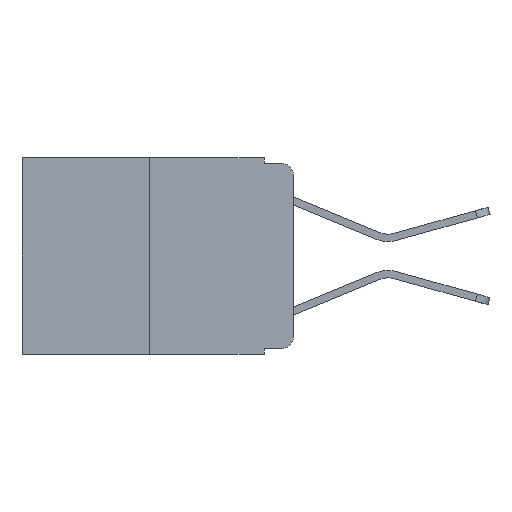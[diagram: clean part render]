
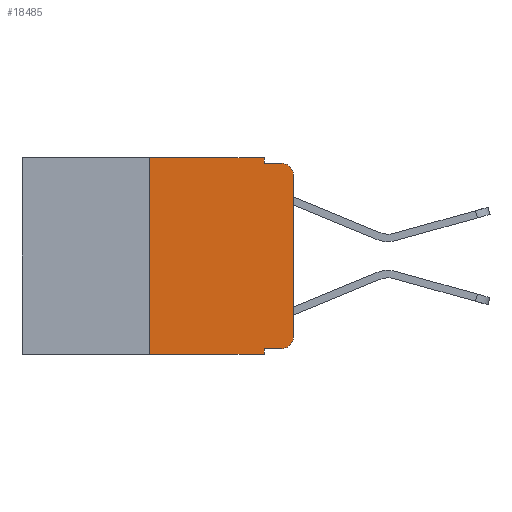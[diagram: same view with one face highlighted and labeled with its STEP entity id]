
A CAD part, left-side view. The second image highlights one B-rep face of the part: STEP entity #18485.
In plain terms, the highlighted planar face has unit normal (-1, 0, 0).
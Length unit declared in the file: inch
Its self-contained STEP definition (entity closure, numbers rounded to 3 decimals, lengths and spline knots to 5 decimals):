
#162 = VECTOR ( 'NONE', #13785, 39.37008 ) ;
#295 = VECTOR ( 'NONE', #14769, 39.37008 ) ;
#560 = VERTEX_POINT ( 'NONE', #21218 ) ;
#864 = EDGE_CURVE ( 'NONE', #19820, #19626, #5667, .T. ) ;
#1301 = LINE ( 'NONE', #9719, #11378 ) ;
#1340 = CARTESIAN_POINT ( 'NONE',  ( 0., 0.051, 0. ) ) ;
#1882 = CARTESIAN_POINT ( 'NONE',  ( 0., 0.051, -0.333 ) ) ;
#2022 = VERTEX_POINT ( 'NONE', #6495 ) ;
#2141 = DIRECTION ( 'NONE',  ( 0., -1., 0. ) ) ;
#2191 = LINE ( 'NONE', #12164, #6284 ) ;
#2541 = AXIS2_PLACEMENT_3D ( 'NONE', #8536, #4469, #12557 ) ;
#3460 = CARTESIAN_POINT ( 'NONE',  ( 0., 0., 0. ) ) ;
#3490 = CARTESIAN_POINT ( 'NONE',  ( 0., 0.25, 0. ) ) ;
#3797 = CARTESIAN_POINT ( 'NONE',  ( 0., 0.051, -0.333 ) ) ;
#3798 = LINE ( 'NONE', #20362, #19010 ) ;
#4059 = LINE ( 'NONE', #1340, #8797 ) ;
#4469 = DIRECTION ( 'NONE',  ( 1., 0., 0. ) ) ;
#4685 = DIRECTION ( 'NONE',  ( 0., -1., 0. ) ) ;
#4912 = EDGE_CURVE ( 'NONE', #14279, #19626, #21799, .T. ) ;
#5306 = FACE_OUTER_BOUND ( 'NONE', #12608, .T. ) ;
#5667 = LINE ( 'NONE', #18038, #295 ) ;
#6263 = EDGE_CURVE ( 'NONE', #2022, #14279, #9125, .T. ) ;
#6284 = VECTOR ( 'NONE', #2141, 39.37008 ) ;
#6495 = CARTESIAN_POINT ( 'NONE',  ( 0., 0., -0.313 ) ) ;
#7077 = CARTESIAN_POINT ( 'NONE',  ( 0., 0.02, -0.333 ) ) ;
#7166 = ORIENTED_EDGE ( 'NONE', *, *, #18697, .T. ) ;
#7593 = DIRECTION ( 'NONE',  ( -1., 0., 0. ) ) ;
#8325 = EDGE_CURVE ( 'NONE', #17697, #23057, #2191, .T. ) ;
#8536 = CARTESIAN_POINT ( 'NONE',  ( 0., 0.473, 0. ) ) ;
#8561 = ORIENTED_EDGE ( 'NONE', *, *, #22612, .F. ) ;
#8695 = ORIENTED_EDGE ( 'NONE', *, *, #6263, .T. ) ;
#8797 = VECTOR ( 'NONE', #17281, 39.37008 ) ;
#9000 = CARTESIAN_POINT ( 'NONE',  ( 0., 0.051, 0. ) ) ;
#9125 = LINE ( 'NONE', #3460, #23536 ) ;
#9307 = DIRECTION ( 'NONE',  ( -1., 0., 0. ) ) ;
#9499 = LINE ( 'NONE', #3490, #18734 ) ;
#9719 = CARTESIAN_POINT ( 'NONE',  ( 0., 0.051, 0. ) ) ;
#9911 = AXIS2_PLACEMENT_3D ( 'NONE', #19409, #7593, #21383 ) ;
#10557 = PLANE ( 'NONE',  #2541 ) ;
#10989 = ORIENTED_EDGE ( 'NONE', *, *, #23901, .F. ) ;
#11378 = VECTOR ( 'NONE', #11750, 39.37008 ) ;
#11750 = DIRECTION ( 'NONE',  ( 0., 0., -1. ) ) ;
#12147 = LINE ( 'NONE', #3797, #162 ) ;
#12164 = CARTESIAN_POINT ( 'NONE',  ( 0., 0.473, 0. ) ) ;
#12557 = DIRECTION ( 'NONE',  ( 0., 0., -1. ) ) ;
#12608 = EDGE_LOOP ( 'NONE', ( #8695, #14910, #12779, #14411, #12871, #10989, #20508, #8561, #22489, #7166 ) ) ;
#12779 = ORIENTED_EDGE ( 'NONE', *, *, #864, .F. ) ;
#12871 = ORIENTED_EDGE ( 'NONE', *, *, #8325, .F. ) ;
#13488 = DIRECTION ( 'NONE',  ( 0., 0., 1. ) ) ;
#13680 = CARTESIAN_POINT ( 'NONE',  ( 0., 0.25, 0. ) ) ;
#13785 = DIRECTION ( 'NONE',  ( 0., -1., 0. ) ) ;
#14052 = CARTESIAN_POINT ( 'NONE',  ( 0., 0., -0.03 ) ) ;
#14279 = VERTEX_POINT ( 'NONE', #14052 ) ;
#14411 = ORIENTED_EDGE ( 'NONE', *, *, #25224, .F. ) ;
#14769 = DIRECTION ( 'NONE',  ( 0., -1., 0. ) ) ;
#14910 = ORIENTED_EDGE ( 'NONE', *, *, #4912, .T. ) ;
#15604 = DIRECTION ( 'NONE',  ( 0., 0., 1. ) ) ;
#17209 = CARTESIAN_POINT ( 'NONE',  ( 0., 0.051, -0.01 ) ) ;
#17281 = DIRECTION ( 'NONE',  ( 0., 0., -1. ) ) ;
#17697 = VERTEX_POINT ( 'NONE', #13680 ) ;
#18038 = CARTESIAN_POINT ( 'NONE',  ( 0., 0.051, -0.01 ) ) ;
#18485 = ADVANCED_FACE ( 'NONE', ( #5306 ), #10557, .F. ) ;
#18697 = EDGE_CURVE ( 'NONE', #25117, #2022, #20766, .T. ) ;
#18734 = VECTOR ( 'NONE', #13488, 39.37008 ) ;
#19010 = VECTOR ( 'NONE', #4685, 39.37008 ) ;
#19409 = CARTESIAN_POINT ( 'NONE',  ( 0., 0.02, -0.03 ) ) ;
#19570 = VERTEX_POINT ( 'NONE', #1882 ) ;
#19626 = VERTEX_POINT ( 'NONE', #19843 ) ;
#19820 = VERTEX_POINT ( 'NONE', #17209 ) ;
#19843 = CARTESIAN_POINT ( 'NONE',  ( 0., 0.02, -0.01 ) ) ;
#20007 = EDGE_CURVE ( 'NONE', #19570, #25117, #12147, .T. ) ;
#20362 = CARTESIAN_POINT ( 'NONE',  ( 0., 0.473, -0.343 ) ) ;
#20508 = ORIENTED_EDGE ( 'NONE', *, *, #22945, .T. ) ;
#20766 = CIRCLE ( 'NONE', #22458, 0.02 ) ;
#21074 = CARTESIAN_POINT ( 'NONE',  ( 0., 0.02, -0.313 ) ) ;
#21218 = CARTESIAN_POINT ( 'NONE',  ( 0., 0.25, -0.343 ) ) ;
#21383 = DIRECTION ( 'NONE',  ( 0., 0., -1. ) ) ;
#21799 = CIRCLE ( 'NONE', #9911, 0.02 ) ;
#22458 = AXIS2_PLACEMENT_3D ( 'NONE', #21074, #9307, #23021 ) ;
#22489 = ORIENTED_EDGE ( 'NONE', *, *, #20007, .T. ) ;
#22612 = EDGE_CURVE ( 'NONE', #19570, #23078, #1301, .T. ) ;
#22945 = EDGE_CURVE ( 'NONE', #560, #23078, #3798, .T. ) ;
#23021 = DIRECTION ( 'NONE',  ( 0., 0., -1. ) ) ;
#23057 = VERTEX_POINT ( 'NONE', #9000 ) ;
#23078 = VERTEX_POINT ( 'NONE', #24772 ) ;
#23536 = VECTOR ( 'NONE', #15604, 39.37008 ) ;
#23901 = EDGE_CURVE ( 'NONE', #560, #17697, #9499, .T. ) ;
#24772 = CARTESIAN_POINT ( 'NONE',  ( 0., 0.051, -0.343 ) ) ;
#25117 = VERTEX_POINT ( 'NONE', #7077 ) ;
#25224 = EDGE_CURVE ( 'NONE', #23057, #19820, #4059, .T. ) ;
